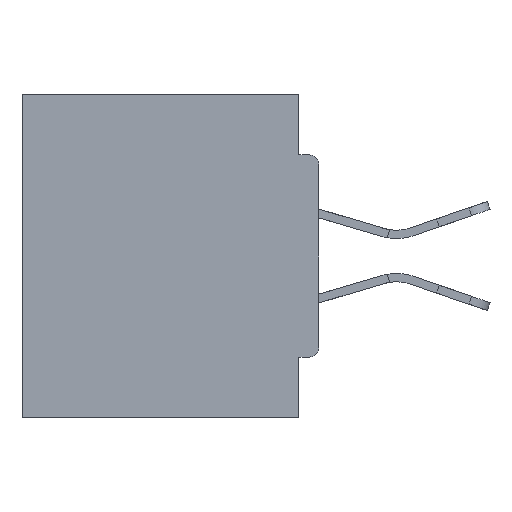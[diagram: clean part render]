
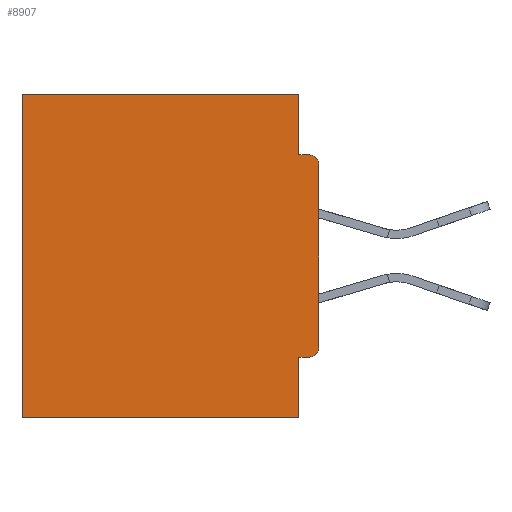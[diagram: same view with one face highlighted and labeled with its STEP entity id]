
A CAD part, left-side view. The second image highlights one B-rep face of the part: STEP entity #8907.
In plain terms, the highlighted planar face has unit normal (-1, 0, 0).
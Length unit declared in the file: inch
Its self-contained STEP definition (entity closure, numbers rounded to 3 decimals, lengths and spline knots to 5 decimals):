
#955 = VECTOR ( 'NONE', #9729, 39.37008 ) ;
#1941 = ORIENTED_EDGE ( 'NONE', *, *, #26245, .F. ) ;
#2040 = DIRECTION ( 'NONE',  ( 1., 0., 0. ) ) ;
#2435 = EDGE_CURVE ( 'NONE', #15353, #13202, #8412, .T. ) ;
#2889 = AXIS2_PLACEMENT_3D ( 'NONE', #22960, #2040, #37806 ) ;
#3764 = EDGE_CURVE ( 'NONE', #7253, #3854, #7451, .T. ) ;
#3854 = VERTEX_POINT ( 'NONE', #5895 ) ;
#4578 = DIRECTION ( 'NONE',  ( 0., 0., -1. ) ) ;
#4936 = CARTESIAN_POINT ( 'NONE',  ( 0.298, 0., 0. ) ) ;
#5761 = ORIENTED_EDGE ( 'NONE', *, *, #31863, .T. ) ;
#5801 = EDGE_LOOP ( 'NONE', ( #5761, #25464, #10174, #30261, #22579, #36665, #21393, #15626, #15710, #1941 ) ) ;
#5895 = CARTESIAN_POINT ( 'NONE',  ( 0.298, 0.46, -0.5 ) ) ;
#5982 = LINE ( 'NONE', #21885, #19727 ) ;
#6442 = DIRECTION ( 'NONE',  ( 0., 0., -1. ) ) ;
#7253 = VERTEX_POINT ( 'NONE', #19927 ) ;
#7451 = LINE ( 'NONE', #31723, #31847 ) ;
#7724 = DIRECTION ( 'NONE',  ( 0., -1., 0. ) ) ;
#8083 = CARTESIAN_POINT ( 'NONE',  ( 0.298, 0.031, -0.5 ) ) ;
#8218 = VERTEX_POINT ( 'NONE', #19647 ) ;
#8412 = CIRCLE ( 'NONE', #37239, 0.015 ) ;
#8623 = EDGE_CURVE ( 'NONE', #15353, #20349, #35048, .T. ) ;
#8907 = ADVANCED_FACE ( 'NONE', ( #13766 ), #37937, .F. ) ;
#9729 = DIRECTION ( 'NONE',  ( 0., 1., 0. ) ) ;
#10174 = ORIENTED_EDGE ( 'NONE', *, *, #10921, .F. ) ;
#10555 = DIRECTION ( 'NONE',  ( 0., 0., -1. ) ) ;
#10757 = CARTESIAN_POINT ( 'NONE',  ( 0.298, 0.031, 0. ) ) ;
#10921 = EDGE_CURVE ( 'NONE', #14383, #8218, #18702, .T. ) ;
#11298 = DIRECTION ( 'NONE',  ( 0., 1., 0. ) ) ;
#11326 = DIRECTION ( 'NONE',  ( -1., 0., 0. ) ) ;
#11696 = DIRECTION ( 'NONE',  ( 0., 0., -1. ) ) ;
#12352 = EDGE_CURVE ( 'NONE', #20349, #30372, #5982, .T. ) ;
#13202 = VERTEX_POINT ( 'NONE', #26629 ) ;
#13744 = CARTESIAN_POINT ( 'NONE',  ( 0.298, 0.015, -0.0935 ) ) ;
#13766 = FACE_OUTER_BOUND ( 'NONE', #5801, .T. ) ;
#14383 = VERTEX_POINT ( 'NONE', #10757 ) ;
#14610 = CARTESIAN_POINT ( 'NONE',  ( 0.298, 0., -0.5 ) ) ;
#15353 = VERTEX_POINT ( 'NONE', #16172 ) ;
#15626 = ORIENTED_EDGE ( 'NONE', *, *, #8623, .F. ) ;
#15710 = ORIENTED_EDGE ( 'NONE', *, *, #2435, .T. ) ;
#16172 = CARTESIAN_POINT ( 'NONE',  ( 0.298, 0.015, -0.4065 ) ) ;
#18157 = CARTESIAN_POINT ( 'NONE',  ( 0.298, 0., -0.1085 ) ) ;
#18702 = LINE ( 'NONE', #32808, #27947 ) ;
#19647 = CARTESIAN_POINT ( 'NONE',  ( 0.298, 0.031, -0.0935 ) ) ;
#19679 = EDGE_CURVE ( 'NONE', #30372, #3854, #22515, .T. ) ;
#19727 = VECTOR ( 'NONE', #4578, 39.37008 ) ;
#19732 = DIRECTION ( 'NONE',  ( 0., 0., -1. ) ) ;
#19927 = CARTESIAN_POINT ( 'NONE',  ( 0.298, 0.46, 0. ) ) ;
#19949 = VECTOR ( 'NONE', #25212, 39.37008 ) ;
#20328 = VECTOR ( 'NONE', #10555, 39.37008 ) ;
#20349 = VERTEX_POINT ( 'NONE', #28869 ) ;
#21393 = ORIENTED_EDGE ( 'NONE', *, *, #12352, .F. ) ;
#21547 = CARTESIAN_POINT ( 'NONE',  ( 0.298, 0., -0.4065 ) ) ;
#21885 = CARTESIAN_POINT ( 'NONE',  ( 0.298, 0.031, -0.5 ) ) ;
#22515 = LINE ( 'NONE', #14610, #23898 ) ;
#22579 = ORIENTED_EDGE ( 'NONE', *, *, #3764, .T. ) ;
#22841 = VERTEX_POINT ( 'NONE', #18157 ) ;
#22960 = CARTESIAN_POINT ( 'NONE',  ( 0.298, 0., 0. ) ) ;
#23116 = LINE ( 'NONE', #25323, #24503 ) ;
#23184 = EDGE_CURVE ( 'NONE', #14383, #7253, #27776, .T. ) ;
#23898 = VECTOR ( 'NONE', #11298, 39.37008 ) ;
#24503 = VECTOR ( 'NONE', #7724, 39.37008 ) ;
#25212 = DIRECTION ( 'NONE',  ( 0., 1., 0. ) ) ;
#25323 = CARTESIAN_POINT ( 'NONE',  ( 0.298, 0., -0.0935 ) ) ;
#25464 = ORIENTED_EDGE ( 'NONE', *, *, #36611, .F. ) ;
#26245 = EDGE_CURVE ( 'NONE', #22841, #13202, #36016, .T. ) ;
#26249 = CIRCLE ( 'NONE', #28780, 0.015 ) ;
#26629 = CARTESIAN_POINT ( 'NONE',  ( 0.298, 0., -0.3915 ) ) ;
#27776 = LINE ( 'NONE', #4936, #19949 ) ;
#27947 = VECTOR ( 'NONE', #6442, 39.37008 ) ;
#28780 = AXIS2_PLACEMENT_3D ( 'NONE', #29441, #11326, #29193 ) ;
#28869 = CARTESIAN_POINT ( 'NONE',  ( 0.298, 0.031, -0.4065 ) ) ;
#29193 = DIRECTION ( 'NONE',  ( 0., 0., -1. ) ) ;
#29315 = DIRECTION ( 'NONE',  ( -1., 0., 0. ) ) ;
#29441 = CARTESIAN_POINT ( 'NONE',  ( 0.298, 0.015, -0.1085 ) ) ;
#30261 = ORIENTED_EDGE ( 'NONE', *, *, #23184, .T. ) ;
#30372 = VERTEX_POINT ( 'NONE', #8083 ) ;
#31723 = CARTESIAN_POINT ( 'NONE',  ( 0.298, 0.46, 0. ) ) ;
#31847 = VECTOR ( 'NONE', #19732, 39.37008 ) ;
#31863 = EDGE_CURVE ( 'NONE', #22841, #33687, #26249, .T. ) ;
#32808 = CARTESIAN_POINT ( 'NONE',  ( 0.298, 0.031, -0.5 ) ) ;
#33687 = VERTEX_POINT ( 'NONE', #13744 ) ;
#33984 = CARTESIAN_POINT ( 'NONE',  ( 0.298, 0., 0. ) ) ;
#35048 = LINE ( 'NONE', #21547, #955 ) ;
#35659 = CARTESIAN_POINT ( 'NONE',  ( 0.298, 0.015, -0.3915 ) ) ;
#36016 = LINE ( 'NONE', #33984, #20328 ) ;
#36611 = EDGE_CURVE ( 'NONE', #8218, #33687, #23116, .T. ) ;
#36665 = ORIENTED_EDGE ( 'NONE', *, *, #19679, .F. ) ;
#37239 = AXIS2_PLACEMENT_3D ( 'NONE', #35659, #29315, #11696 ) ;
#37806 = DIRECTION ( 'NONE',  ( 0., 0., -1. ) ) ;
#37937 = PLANE ( 'NONE',  #2889 ) ;
